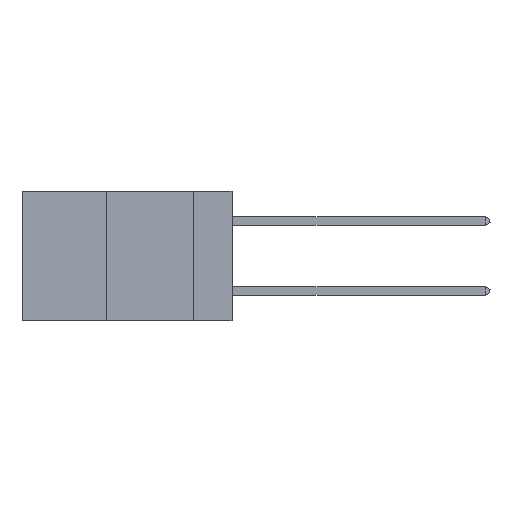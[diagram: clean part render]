
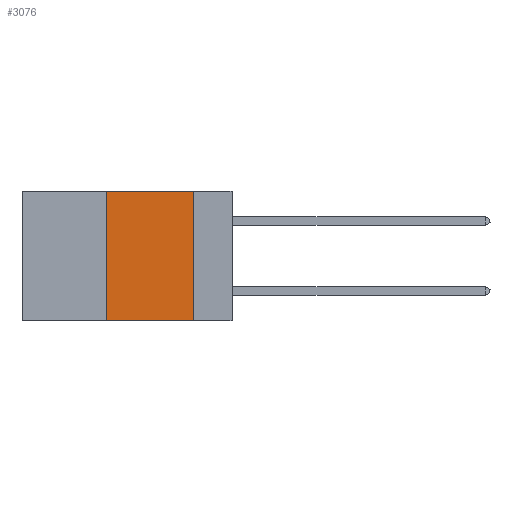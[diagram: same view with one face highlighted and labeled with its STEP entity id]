
A CAD part, left-side view. The second image highlights one B-rep face of the part: STEP entity #3076.
In plain terms, the highlighted planar face has unit normal (-1, 0, 0).
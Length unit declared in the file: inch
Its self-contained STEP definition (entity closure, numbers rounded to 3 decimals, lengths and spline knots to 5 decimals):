
#427 = CARTESIAN_POINT ( 'NONE',  ( 0., 0.11, 0. ) ) ;
#912 = VECTOR ( 'NONE', #16931, 39.37008 ) ;
#3076 = ADVANCED_FACE ( 'NONE', ( #32233 ), #29483, .F. ) ;
#4109 = VERTEX_POINT ( 'NONE', #22119 ) ;
#7018 = DIRECTION ( 'NONE',  ( 1., 0., 0. ) ) ;
#8022 = ORIENTED_EDGE ( 'NONE', *, *, #31421, .T. ) ;
#8913 = CARTESIAN_POINT ( 'NONE',  ( 0., 0.6, 0. ) ) ;
#11685 = VECTOR ( 'NONE', #15163, 39.37008 ) ;
#12454 = VECTOR ( 'NONE', #29270, 39.37008 ) ;
#13526 = CARTESIAN_POINT ( 'NONE',  ( 0., 0.6, -0.37 ) ) ;
#13591 = VERTEX_POINT ( 'NONE', #24406 ) ;
#14249 = AXIS2_PLACEMENT_3D ( 'NONE', #29349, #7018, #32612 ) ;
#15163 = DIRECTION ( 'NONE',  ( 0., -1., 0. ) ) ;
#15617 = CARTESIAN_POINT ( 'NONE',  ( 0., 0.36, -0.37 ) ) ;
#15628 = EDGE_CURVE ( 'NONE', #4109, #38467, #19316, .T. ) ;
#16931 = DIRECTION ( 'NONE',  ( 0., -1., 0. ) ) ;
#19316 = LINE ( 'NONE', #8913, #11685 ) ;
#19630 = LINE ( 'NONE', #427, #29862 ) ;
#20049 = DIRECTION ( 'NONE',  ( 0., 0., -1. ) ) ;
#21109 = LINE ( 'NONE', #39244, #12454 ) ;
#22119 = CARTESIAN_POINT ( 'NONE',  ( 0., 0.36, 0. ) ) ;
#24406 = CARTESIAN_POINT ( 'NONE',  ( 0., 0.11, -0.37 ) ) ;
#25646 = ORIENTED_EDGE ( 'NONE', *, *, #38989, .F. ) ;
#26859 = LINE ( 'NONE', #13526, #912 ) ;
#29270 = DIRECTION ( 'NONE',  ( 0., 0., 1. ) ) ;
#29349 = CARTESIAN_POINT ( 'NONE',  ( 0., 0.6, 0. ) ) ;
#29483 = PLANE ( 'NONE',  #14249 ) ;
#29862 = VECTOR ( 'NONE', #20049, 39.37008 ) ;
#31421 = EDGE_CURVE ( 'NONE', #37619, #13591, #26859, .T. ) ;
#32233 = FACE_OUTER_BOUND ( 'NONE', #33647, .T. ) ;
#32612 = DIRECTION ( 'NONE',  ( 0., 0., -1. ) ) ;
#33616 = CARTESIAN_POINT ( 'NONE',  ( 0., 0.11, 0. ) ) ;
#33647 = EDGE_LOOP ( 'NONE', ( #25646, #36715, #40969, #8022 ) ) ;
#36715 = ORIENTED_EDGE ( 'NONE', *, *, #15628, .F. ) ;
#37619 = VERTEX_POINT ( 'NONE', #15617 ) ;
#38467 = VERTEX_POINT ( 'NONE', #33616 ) ;
#38989 = EDGE_CURVE ( 'NONE', #38467, #13591, #19630, .T. ) ;
#39244 = CARTESIAN_POINT ( 'NONE',  ( 0., 0.36, 0. ) ) ;
#39577 = EDGE_CURVE ( 'NONE', #37619, #4109, #21109, .T. ) ;
#40969 = ORIENTED_EDGE ( 'NONE', *, *, #39577, .F. ) ;
